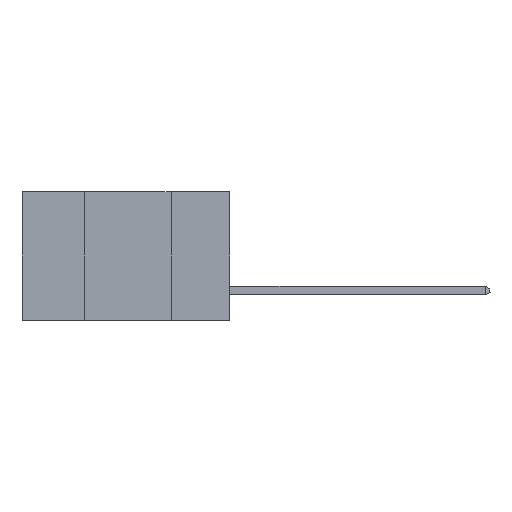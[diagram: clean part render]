
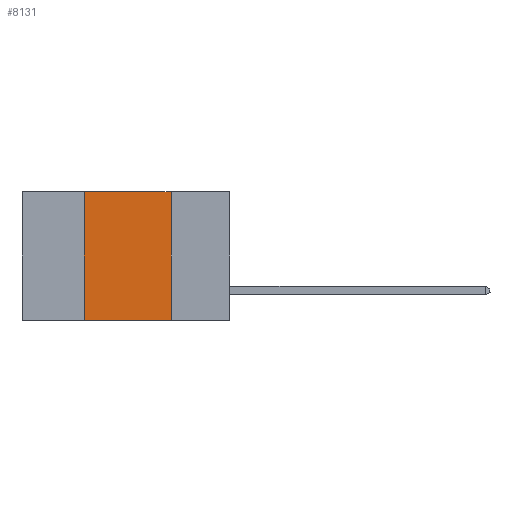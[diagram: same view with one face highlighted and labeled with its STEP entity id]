
A CAD part, left-side view. The second image highlights one B-rep face of the part: STEP entity #8131.
In plain terms, the highlighted planar face has unit normal (-1, 0, 0).
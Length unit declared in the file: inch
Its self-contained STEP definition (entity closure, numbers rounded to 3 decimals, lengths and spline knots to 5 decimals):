
#5 = LINE ( 'NONE', #3773, #3691 ) ;
#264 = ORIENTED_EDGE ( 'NONE', *, *, #6799, .F. ) ;
#571 = LINE ( 'NONE', #754, #6154 ) ;
#754 = CARTESIAN_POINT ( 'NONE',  ( 0., 0.6, 0. ) ) ;
#1099 = CARTESIAN_POINT ( 'NONE',  ( 0., 0.42, -0.37 ) ) ;
#1571 = CARTESIAN_POINT ( 'NONE',  ( 0., 0.42, 0. ) ) ;
#1619 = DIRECTION ( 'NONE',  ( 0., 0., -1. ) ) ;
#1698 = CARTESIAN_POINT ( 'NONE',  ( 0., 0.6, -0.37 ) ) ;
#1763 = DIRECTION ( 'NONE',  ( 0., 0., 1. ) ) ;
#2816 = EDGE_CURVE ( 'NONE', #5821, #7265, #9639, .T. ) ;
#2817 = ORIENTED_EDGE ( 'NONE', *, *, #4312, .F. ) ;
#3691 = VECTOR ( 'NONE', #1763, 39.37008 ) ;
#3773 = CARTESIAN_POINT ( 'NONE',  ( 0., 0.42, 0. ) ) ;
#3784 = VERTEX_POINT ( 'NONE', #1571 ) ;
#3817 = VECTOR ( 'NONE', #10328, 39.37008 ) ;
#4312 = EDGE_CURVE ( 'NONE', #3784, #5821, #571, .T. ) ;
#5733 = CARTESIAN_POINT ( 'NONE',  ( 0., 0.17, -0.37 ) ) ;
#5821 = VERTEX_POINT ( 'NONE', #7194 ) ;
#6154 = VECTOR ( 'NONE', #10489, 39.37008 ) ;
#6660 = DIRECTION ( 'NONE',  ( 1., 0., 0. ) ) ;
#6799 = EDGE_CURVE ( 'NONE', #13051, #3784, #5, .T. ) ;
#6829 = AXIS2_PLACEMENT_3D ( 'NONE', #12917, #6660, #1619 ) ;
#7194 = CARTESIAN_POINT ( 'NONE',  ( 0., 0.17, 0. ) ) ;
#7265 = VERTEX_POINT ( 'NONE', #5733 ) ;
#7467 = VECTOR ( 'NONE', #9746, 39.37008 ) ;
#8129 = LINE ( 'NONE', #1698, #7467 ) ;
#8131 = ADVANCED_FACE ( 'NONE', ( #9313 ), #9905, .F. ) ;
#8436 = EDGE_CURVE ( 'NONE', #13051, #7265, #8129, .T. ) ;
#8598 = ORIENTED_EDGE ( 'NONE', *, *, #2816, .F. ) ;
#9313 = FACE_OUTER_BOUND ( 'NONE', #9982, .T. ) ;
#9639 = LINE ( 'NONE', #13364, #3817 ) ;
#9746 = DIRECTION ( 'NONE',  ( 0., -1., 0. ) ) ;
#9905 = PLANE ( 'NONE',  #6829 ) ;
#9982 = EDGE_LOOP ( 'NONE', ( #8598, #2817, #264, #11788 ) ) ;
#10328 = DIRECTION ( 'NONE',  ( 0., 0., -1. ) ) ;
#10489 = DIRECTION ( 'NONE',  ( 0., -1., 0. ) ) ;
#11788 = ORIENTED_EDGE ( 'NONE', *, *, #8436, .T. ) ;
#12917 = CARTESIAN_POINT ( 'NONE',  ( 0., 0.6, 0. ) ) ;
#13051 = VERTEX_POINT ( 'NONE', #1099 ) ;
#13364 = CARTESIAN_POINT ( 'NONE',  ( 0., 0.17, 0. ) ) ;
